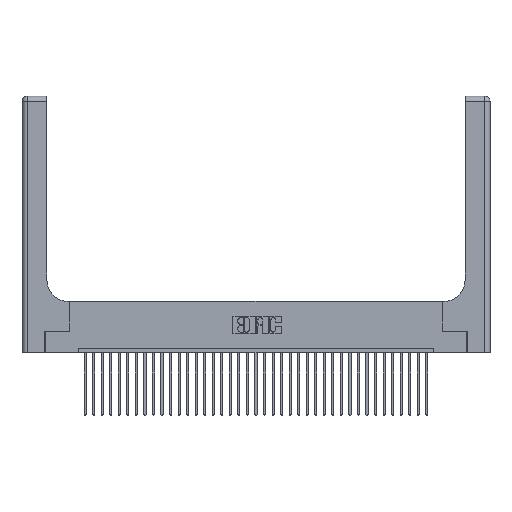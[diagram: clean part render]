
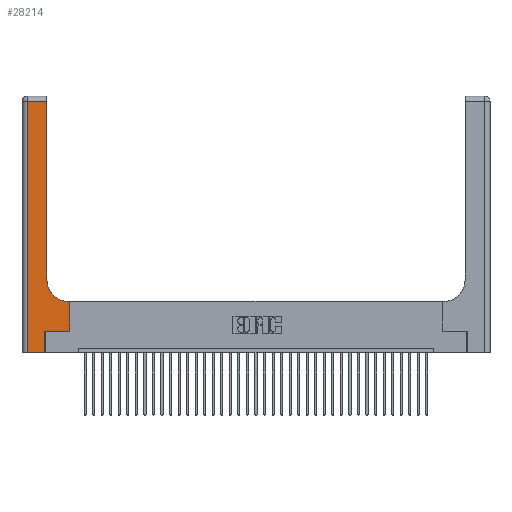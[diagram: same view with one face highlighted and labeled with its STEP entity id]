
A CAD part, top view. The second image highlights one B-rep face of the part: STEP entity #28214.
In plain terms, the highlighted planar face has unit normal (0, 0, 1).
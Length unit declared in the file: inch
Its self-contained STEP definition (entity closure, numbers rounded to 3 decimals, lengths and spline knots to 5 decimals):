
#128 = DIRECTION ( 'NONE',  ( -1., 0., 0. ) ) ;
#1180 = LINE ( 'NONE', #9970, #19475 ) ;
#1330 = VECTOR ( 'NONE', #28431, 39.37008 ) ;
#1544 = CARTESIAN_POINT ( 'NONE',  ( 0., 0., 0.37 ) ) ;
#1597 = CARTESIAN_POINT ( 'NONE',  ( 0.2915, 2.94, 0.37 ) ) ;
#1610 = EDGE_CURVE ( 'NONE', #24567, #32883, #30732, .T. ) ;
#2415 = ORIENTED_EDGE ( 'NONE', *, *, #1610, .T. ) ;
#2922 = LINE ( 'NONE', #8881, #1330 ) ;
#3367 = AXIS2_PLACEMENT_3D ( 'NONE', #18152, #15365, #9755 ) ;
#3376 = EDGE_CURVE ( 'NONE', #5451, #21088, #15239, .T. ) ;
#4144 = ORIENTED_EDGE ( 'NONE', *, *, #5930, .T. ) ;
#4200 = CARTESIAN_POINT ( 'NONE',  ( 0.06, 3., 0.37 ) ) ;
#5451 = VERTEX_POINT ( 'NONE', #32508 ) ;
#5930 = EDGE_CURVE ( 'NONE', #26602, #10130, #32197, .T. ) ;
#6200 = VECTOR ( 'NONE', #6978, 39.37008 ) ;
#6402 = ORIENTED_EDGE ( 'NONE', *, *, #12210, .T. ) ;
#6978 = DIRECTION ( 'NONE',  ( 0., -1., 0. ) ) ;
#7092 = CARTESIAN_POINT ( 'NONE',  ( 0.269, 0.25, 0.37 ) ) ;
#8678 = CARTESIAN_POINT ( 'NONE',  ( 0.5415, 0.6, 0.37 ) ) ;
#8824 = LINE ( 'NONE', #4200, #6200 ) ;
#8881 = CARTESIAN_POINT ( 'NONE',  ( 0., 2.94, 0.37 ) ) ;
#9363 = VERTEX_POINT ( 'NONE', #28656 ) ;
#9755 = DIRECTION ( 'NONE',  ( 1., 0., 0. ) ) ;
#9834 = DIRECTION ( 'NONE',  ( 0., 1., 0. ) ) ;
#9970 = CARTESIAN_POINT ( 'NONE',  ( 0.2915, 3., 0.37 ) ) ;
#10130 = VERTEX_POINT ( 'NONE', #25469 ) ;
#10835 = LINE ( 'NONE', #1544, #36199 ) ;
#12210 = EDGE_CURVE ( 'NONE', #9363, #16475, #8824, .T. ) ;
#12349 = CARTESIAN_POINT ( 'NONE',  ( 0.5585, 0.25, 0.37 ) ) ;
#12462 = ORIENTED_EDGE ( 'NONE', *, *, #20810, .T. ) ;
#12759 = DIRECTION ( 'NONE',  ( 1., 0., 0. ) ) ;
#13100 = PLANE ( 'NONE',  #34596 ) ;
#14098 = CARTESIAN_POINT ( 'NONE',  ( 0.269, 0.25, 0.37 ) ) ;
#14504 = CARTESIAN_POINT ( 'NONE',  ( 0.5585, 0.25, 0.37 ) ) ;
#14803 = ORIENTED_EDGE ( 'NONE', *, *, #18968, .T. ) ;
#15239 = LINE ( 'NONE', #17635, #16542 ) ;
#15365 = DIRECTION ( 'NONE',  ( 0., 0., -1. ) ) ;
#15984 = DIRECTION ( 'NONE',  ( -1., 0., 0. ) ) ;
#16197 = EDGE_CURVE ( 'NONE', #16475, #5451, #10835, .T. ) ;
#16475 = VERTEX_POINT ( 'NONE', #21861 ) ;
#16542 = VECTOR ( 'NONE', #20574, 39.37008 ) ;
#17259 = VECTOR ( 'NONE', #128, 39.37008 ) ;
#17635 = CARTESIAN_POINT ( 'NONE',  ( 0.269, 0., 0.37 ) ) ;
#17790 = VERTEX_POINT ( 'NONE', #1597 ) ;
#18152 = CARTESIAN_POINT ( 'NONE',  ( 0.5415, 0.85, 0.37 ) ) ;
#18248 = LINE ( 'NONE', #7092, #27886 ) ;
#18878 = VECTOR ( 'NONE', #9834, 39.37008 ) ;
#18968 = EDGE_CURVE ( 'NONE', #21088, #24567, #18248, .T. ) ;
#19217 = FACE_OUTER_BOUND ( 'NONE', #25803, .T. ) ;
#19475 = VECTOR ( 'NONE', #35168, 39.37008 ) ;
#19484 = CARTESIAN_POINT ( 'NONE',  ( 0.2915, 0.6, 0.37 ) ) ;
#20574 = DIRECTION ( 'NONE',  ( 0., 1., 0. ) ) ;
#20810 = EDGE_CURVE ( 'NONE', #10130, #17790, #1180, .T. ) ;
#21088 = VERTEX_POINT ( 'NONE', #14098 ) ;
#21861 = CARTESIAN_POINT ( 'NONE',  ( 0.06, 0., 0.37 ) ) ;
#22244 = ORIENTED_EDGE ( 'NONE', *, *, #31621, .T. ) ;
#22670 = CARTESIAN_POINT ( 'NONE',  ( 0.5585, 0.6, 0.37 ) ) ;
#24450 = ORIENTED_EDGE ( 'NONE', *, *, #16197, .T. ) ;
#24567 = VERTEX_POINT ( 'NONE', #12349 ) ;
#25315 = ORIENTED_EDGE ( 'NONE', *, *, #3376, .T. ) ;
#25469 = CARTESIAN_POINT ( 'NONE',  ( 0.2915, 0.85, 0.37 ) ) ;
#25803 = EDGE_LOOP ( 'NONE', ( #12462, #32266, #6402, #24450, #25315, #14803, #2415, #22244, #4144 ) ) ;
#26602 = VERTEX_POINT ( 'NONE', #8678 ) ;
#26905 = DIRECTION ( 'NONE',  ( 1., 0., 0. ) ) ;
#27886 = VECTOR ( 'NONE', #26905, 39.37008 ) ;
#28214 = ADVANCED_FACE ( 'NONE', ( #19217 ), #13100, .F. ) ;
#28431 = DIRECTION ( 'NONE',  ( -1., 0., 0. ) ) ;
#28656 = CARTESIAN_POINT ( 'NONE',  ( 0.06, 2.94, 0.37 ) ) ;
#30732 = LINE ( 'NONE', #14504, #18878 ) ;
#31621 = EDGE_CURVE ( 'NONE', #32883, #26602, #33064, .T. ) ;
#32197 = CIRCLE ( 'NONE', #3367, 0.25 ) ;
#32266 = ORIENTED_EDGE ( 'NONE', *, *, #34723, .T. ) ;
#32301 = DIRECTION ( 'NONE',  ( 0., 0., -1. ) ) ;
#32508 = CARTESIAN_POINT ( 'NONE',  ( 0.269, 0., 0.37 ) ) ;
#32546 = CARTESIAN_POINT ( 'NONE',  ( 0., 3., 0.37 ) ) ;
#32883 = VERTEX_POINT ( 'NONE', #22670 ) ;
#33064 = LINE ( 'NONE', #19484, #17259 ) ;
#34596 = AXIS2_PLACEMENT_3D ( 'NONE', #32546, #32301, #15984 ) ;
#34723 = EDGE_CURVE ( 'NONE', #17790, #9363, #2922, .T. ) ;
#35168 = DIRECTION ( 'NONE',  ( 0., 1., 0. ) ) ;
#36199 = VECTOR ( 'NONE', #12759, 39.37008 ) ;
